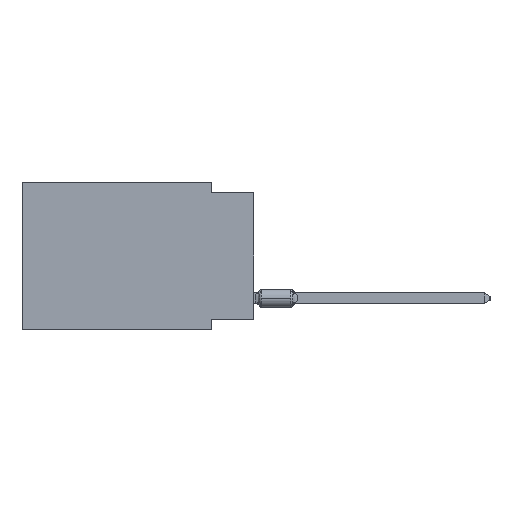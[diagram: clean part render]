
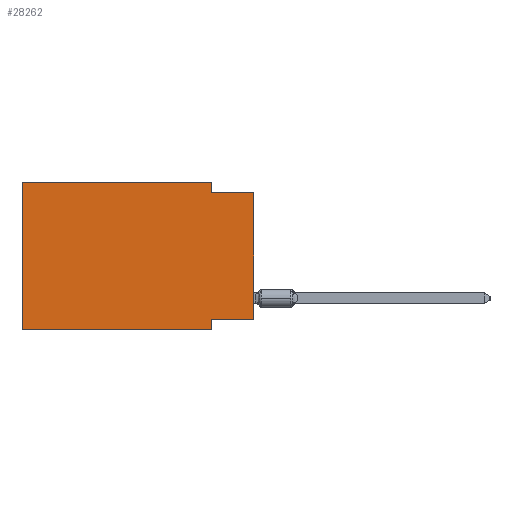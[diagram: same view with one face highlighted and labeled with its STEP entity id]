
A CAD part, left-side view. The second image highlights one B-rep face of the part: STEP entity #28262.
In plain terms, the highlighted planar face has unit normal (-1, 0, 0).
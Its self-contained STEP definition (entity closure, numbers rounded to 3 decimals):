
#1360 = LINE ( 'NONE', #34845, #30704 ) ;
#1539 = LINE ( 'NONE', #59447, #46358 ) ;
#3297 = EDGE_CURVE ( 'NONE', #63089, #52660, #11176, .T. ) ;
#4128 = EDGE_CURVE ( 'NONE', #44554, #63089, #59453, .T. ) ;
#4572 = AXIS2_PLACEMENT_3D ( 'NONE', #32551, #14304, #60804 ) ;
#9551 = VECTOR ( 'NONE', #21574, 1000. ) ;
#10964 = DIRECTION ( 'NONE',  ( 0., -1., 0. ) ) ;
#11176 = LINE ( 'NONE', #69481, #29342 ) ;
#11834 = VERTEX_POINT ( 'NONE', #27787 ) ;
#13352 = VERTEX_POINT ( 'NONE', #72729 ) ;
#14304 = DIRECTION ( 'NONE',  ( 1., 0., 0. ) ) ;
#14571 = ORIENTED_EDGE ( 'NONE', *, *, #42550, .F. ) ;
#16878 = DIRECTION ( 'NONE',  ( 0., -1., 0. ) ) ;
#16964 = ORIENTED_EDGE ( 'NONE', *, *, #69339, .T. ) ;
#20146 = DIRECTION ( 'NONE',  ( 0., 0., 1. ) ) ;
#20294 = VECTOR ( 'NONE', #26867, 1000. ) ;
#20371 = ORIENTED_EDGE ( 'NONE', *, *, #42343, .F. ) ;
#21574 = DIRECTION ( 'NONE',  ( 0., 1., 0. ) ) ;
#24742 = DIRECTION ( 'NONE',  ( 0., -1., 0. ) ) ;
#25068 = VERTEX_POINT ( 'NONE', #29780 ) ;
#26256 = CARTESIAN_POINT ( 'NONE',  ( 0., 13.97, -8.89 ) ) ;
#26867 = DIRECTION ( 'NONE',  ( 0., 0., -1. ) ) ;
#27236 = CARTESIAN_POINT ( 'NONE',  ( 0., 2.54, -8.89 ) ) ;
#27787 = CARTESIAN_POINT ( 'NONE',  ( 0., 0., -8.255 ) ) ;
#28262 = ADVANCED_FACE ( 'NONE', ( #31059 ), #72999, .F. ) ;
#28832 = ORIENTED_EDGE ( 'NONE', *, *, #59616, .F. ) ;
#29342 = VECTOR ( 'NONE', #16878, 1000. ) ;
#29780 = CARTESIAN_POINT ( 'NONE',  ( 0., 2.54, -8.89 ) ) ;
#30134 = ORIENTED_EDGE ( 'NONE', *, *, #70180, .T. ) ;
#30704 = VECTOR ( 'NONE', #42092, 1000. ) ;
#30810 = ORIENTED_EDGE ( 'NONE', *, *, #3297, .F. ) ;
#31059 = FACE_OUTER_BOUND ( 'NONE', #32129, .T. ) ;
#32129 = EDGE_LOOP ( 'NONE', ( #30134, #30810, #54143, #14571, #20371, #16964, #57426, #28832 ) ) ;
#32551 = CARTESIAN_POINT ( 'NONE',  ( 0., 13.97, 0. ) ) ;
#33385 = CARTESIAN_POINT ( 'NONE',  ( 0., 0., -8.255 ) ) ;
#34845 = CARTESIAN_POINT ( 'NONE',  ( 0., 0., 0. ) ) ;
#38627 = VECTOR ( 'NONE', #20146, 1000. ) ;
#42092 = DIRECTION ( 'NONE',  ( 0., 0., 1. ) ) ;
#42343 = EDGE_CURVE ( 'NONE', #61169, #13352, #43378, .T. ) ;
#42550 = EDGE_CURVE ( 'NONE', #13352, #44554, #58210, .T. ) ;
#43378 = LINE ( 'NONE', #60939, #38627 ) ;
#44554 = VERTEX_POINT ( 'NONE', #59623 ) ;
#44838 = LINE ( 'NONE', #33385, #9551 ) ;
#45418 = CARTESIAN_POINT ( 'NONE',  ( 0., 0., -0.635 ) ) ;
#46358 = VECTOR ( 'NONE', #24742, 1000. ) ;
#48765 = DIRECTION ( 'NONE',  ( 0., 0., -1. ) ) ;
#52112 = CARTESIAN_POINT ( 'NONE',  ( 0., 13.97, 0. ) ) ;
#52660 = VERTEX_POINT ( 'NONE', #45418 ) ;
#52719 = CARTESIAN_POINT ( 'NONE',  ( 0., 2.54, -0.635 ) ) ;
#53934 = VERTEX_POINT ( 'NONE', #69415 ) ;
#54111 = CARTESIAN_POINT ( 'NONE',  ( 0., 2.54, 0. ) ) ;
#54143 = ORIENTED_EDGE ( 'NONE', *, *, #4128, .F. ) ;
#57426 = ORIENTED_EDGE ( 'NONE', *, *, #73077, .F. ) ;
#58210 = LINE ( 'NONE', #52112, #71591 ) ;
#59447 = CARTESIAN_POINT ( 'NONE',  ( 0., 13.97, -8.89 ) ) ;
#59453 = LINE ( 'NONE', #54111, #70857 ) ;
#59616 = EDGE_CURVE ( 'NONE', #11834, #53934, #44838, .T. ) ;
#59623 = CARTESIAN_POINT ( 'NONE',  ( 0., 2.54, 0. ) ) ;
#60804 = DIRECTION ( 'NONE',  ( 0., 0., -1. ) ) ;
#60939 = CARTESIAN_POINT ( 'NONE',  ( 0., 13.97, 0. ) ) ;
#61169 = VERTEX_POINT ( 'NONE', #26256 ) ;
#61938 = LINE ( 'NONE', #27236, #20294 ) ;
#63089 = VERTEX_POINT ( 'NONE', #52719 ) ;
#69339 = EDGE_CURVE ( 'NONE', #61169, #25068, #1539, .T. ) ;
#69415 = CARTESIAN_POINT ( 'NONE',  ( 0., 2.54, -8.255 ) ) ;
#69481 = CARTESIAN_POINT ( 'NONE',  ( 0., 0., -0.635 ) ) ;
#70180 = EDGE_CURVE ( 'NONE', #11834, #52660, #1360, .T. ) ;
#70857 = VECTOR ( 'NONE', #48765, 1000. ) ;
#71591 = VECTOR ( 'NONE', #10964, 1000. ) ;
#72729 = CARTESIAN_POINT ( 'NONE',  ( 0., 13.97, 0. ) ) ;
#72999 = PLANE ( 'NONE',  #4572 ) ;
#73077 = EDGE_CURVE ( 'NONE', #53934, #25068, #61938, .T. ) ;
